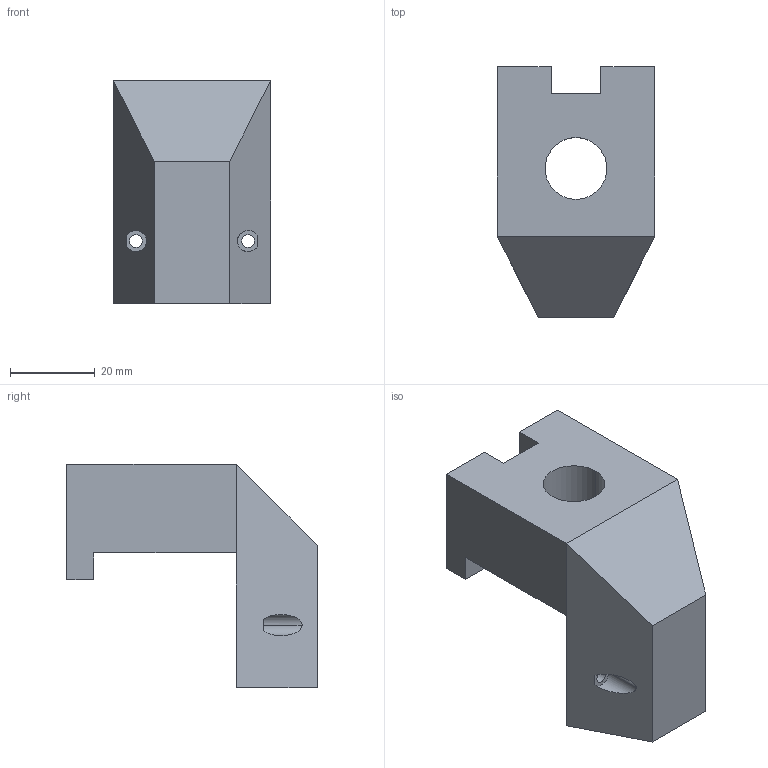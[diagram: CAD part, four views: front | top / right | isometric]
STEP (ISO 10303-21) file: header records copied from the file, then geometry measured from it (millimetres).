
FILE_DESCRIPTION (( 'STEP AP214' ), '1' );
FILE_NAME ('BARREL_RETAINER.STEP', '2013-05-15T15:06:22', ( 'Asher' ), ( '' ), 'SwSTEP 2.0', 'SolidWorks 2013', '' );
FILE_SCHEMA (( 'AUTOMOTIVE_DESIGN' ));
Length unit declared in the file: inch
Products named in the file (1): BARREL_RETAINER
Bounding box: 37.08 x 59.05 x 52.58 mm (x, y, z)
Volume: 48866.4 mm3; surface area: 11841.7 mm2
Topology: 1 solids, 1 shells, 35 faces, 84 edges, 54 vertices
Faces by surface type: plane 26, cylinder 9
Entity records: 1060 total; most frequent: CARTESIAN_POINT 186, DIRECTION 168, ORIENTED_EDGE 168, EDGE_CURVE 84, VECTOR 66, LINE 66, VERTEX_POINT 54, AXIS2_PLACEMENT_3D 51
